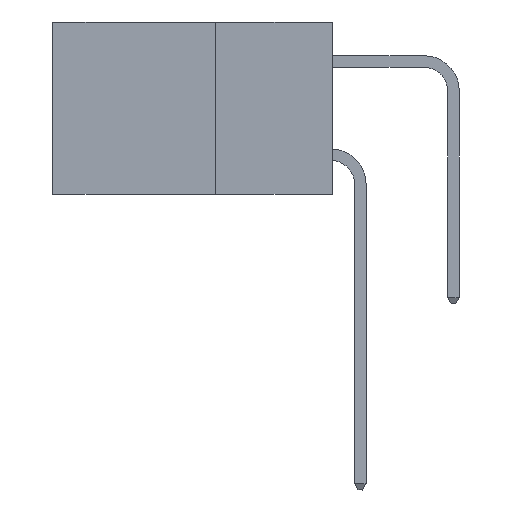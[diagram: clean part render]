
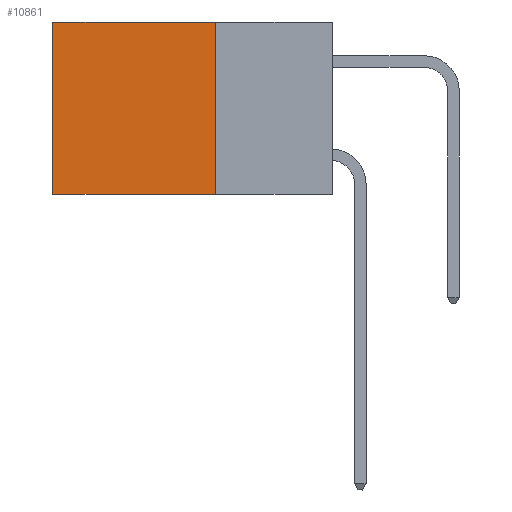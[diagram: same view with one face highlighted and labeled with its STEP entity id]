
A CAD part, left-side view. The second image highlights one B-rep face of the part: STEP entity #10861.
In plain terms, the highlighted planar face has unit normal (-1, 0, 0).
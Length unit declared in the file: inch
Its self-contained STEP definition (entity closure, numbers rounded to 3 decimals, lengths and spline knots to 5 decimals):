
#1818 = CARTESIAN_POINT ( 'NONE',  ( 0.298, 0.6, 0. ) ) ;
#2529 = DIRECTION ( 'NONE',  ( 0., 0., -1. ) ) ;
#2649 = CARTESIAN_POINT ( 'NONE',  ( 0.298, 0.25, -0.37 ) ) ;
#3352 = EDGE_CURVE ( 'NONE', #15082, #14407, #15927, .T. ) ;
#3697 = ORIENTED_EDGE ( 'NONE', *, *, #16518, .F. ) ;
#4770 = ORIENTED_EDGE ( 'NONE', *, *, #4775, .T. ) ;
#4775 = EDGE_CURVE ( 'NONE', #16189, #14407, #15885, .T. ) ;
#4994 = FACE_OUTER_BOUND ( 'NONE', #19592, .T. ) ;
#5200 = CARTESIAN_POINT ( 'NONE',  ( 0.298, 0.25, 0. ) ) ;
#6931 = CARTESIAN_POINT ( 'NONE',  ( 0.298, 0.25, 0. ) ) ;
#9651 = VERTEX_POINT ( 'NONE', #6931 ) ;
#10861 = ADVANCED_FACE ( 'NONE', ( #4994 ), #12857, .F. ) ;
#11934 = AXIS2_PLACEMENT_3D ( 'NONE', #18205, #23775, #20150 ) ;
#11943 = CARTESIAN_POINT ( 'NONE',  ( 0.298, 0.6, 0. ) ) ;
#12857 = PLANE ( 'NONE',  #11934 ) ;
#12942 = CARTESIAN_POINT ( 'NONE',  ( 0.298, 0.6, -0.37 ) ) ;
#13029 = EDGE_CURVE ( 'NONE', #9651, #16189, #20174, .T. ) ;
#14346 = CARTESIAN_POINT ( 'NONE',  ( 0.298, 0.25, 0. ) ) ;
#14407 = VERTEX_POINT ( 'NONE', #12942 ) ;
#14532 = DIRECTION ( 'NONE',  ( 0., 1., 0. ) ) ;
#15082 = VERTEX_POINT ( 'NONE', #16034 ) ;
#15836 = VECTOR ( 'NONE', #14532, 39.37008 ) ;
#15885 = LINE ( 'NONE', #1818, #19947 ) ;
#15927 = LINE ( 'NONE', #2649, #22294 ) ;
#16034 = CARTESIAN_POINT ( 'NONE',  ( 0.298, 0.25, -0.37 ) ) ;
#16189 = VERTEX_POINT ( 'NONE', #11943 ) ;
#16518 = EDGE_CURVE ( 'NONE', #9651, #15082, #23739, .T. ) ;
#17392 = VECTOR ( 'NONE', #21886, 39.37008 ) ;
#18205 = CARTESIAN_POINT ( 'NONE',  ( 0.298, 0.25, 0. ) ) ;
#18264 = ORIENTED_EDGE ( 'NONE', *, *, #13029, .T. ) ;
#19592 = EDGE_LOOP ( 'NONE', ( #4770, #22512, #3697, #18264 ) ) ;
#19947 = VECTOR ( 'NONE', #2529, 39.37008 ) ;
#20150 = DIRECTION ( 'NONE',  ( 0., 0., -1. ) ) ;
#20174 = LINE ( 'NONE', #5200, #15836 ) ;
#21488 = DIRECTION ( 'NONE',  ( 0., 1., 0. ) ) ;
#21886 = DIRECTION ( 'NONE',  ( 0., 0., -1. ) ) ;
#22294 = VECTOR ( 'NONE', #21488, 39.37008 ) ;
#22512 = ORIENTED_EDGE ( 'NONE', *, *, #3352, .F. ) ;
#23739 = LINE ( 'NONE', #14346, #17392 ) ;
#23775 = DIRECTION ( 'NONE',  ( 1., 0., 0. ) ) ;
